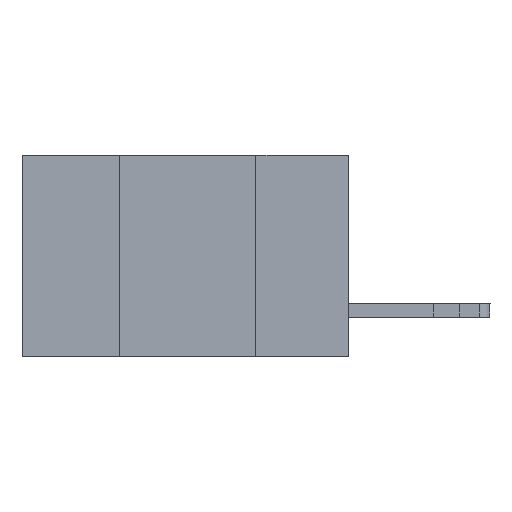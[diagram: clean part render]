
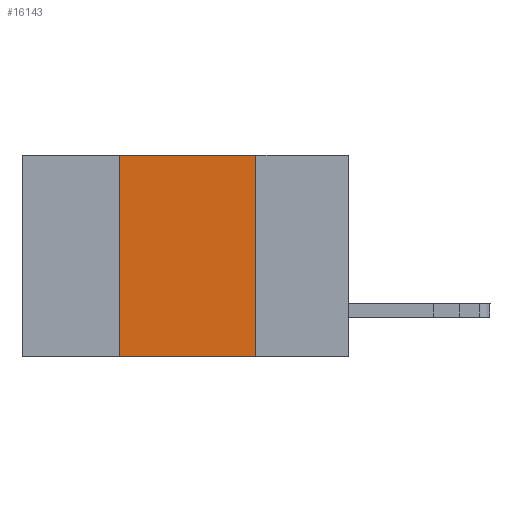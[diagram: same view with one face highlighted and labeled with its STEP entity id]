
A CAD part, left-side view. The second image highlights one B-rep face of the part: STEP entity #16143.
In plain terms, the highlighted planar face has unit normal (-1, 0, 0).
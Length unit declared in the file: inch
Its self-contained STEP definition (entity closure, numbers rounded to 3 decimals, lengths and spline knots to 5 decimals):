
#485 = AXIS2_PLACEMENT_3D ( 'NONE', #12607, #7604, #16830 ) ;
#1100 = EDGE_CURVE ( 'NONE', #4532, #9982, #6542, .T. ) ;
#1415 = ORIENTED_EDGE ( 'NONE', *, *, #6935, .F. ) ;
#1929 = VERTEX_POINT ( 'NONE', #5310 ) ;
#2057 = LINE ( 'NONE', #10616, #3103 ) ;
#2559 = LINE ( 'NONE', #4682, #4632 ) ;
#3103 = VECTOR ( 'NONE', #12013, 39.37008 ) ;
#3116 = EDGE_CURVE ( 'NONE', #1929, #9982, #2057, .T. ) ;
#3257 = LINE ( 'NONE', #12045, #14422 ) ;
#3979 = EDGE_LOOP ( 'NONE', ( #4754, #1415, #14849, #15293 ) ) ;
#4532 = VERTEX_POINT ( 'NONE', #10554 ) ;
#4632 = VECTOR ( 'NONE', #11650, 39.37008 ) ;
#4682 = CARTESIAN_POINT ( 'NONE',  ( 0., 0.6, 0. ) ) ;
#4754 = ORIENTED_EDGE ( 'NONE', *, *, #3116, .F. ) ;
#5310 = CARTESIAN_POINT ( 'NONE',  ( 0., 0.17, 0. ) ) ;
#6336 = CARTESIAN_POINT ( 'NONE',  ( 0., 0.17, -0.37 ) ) ;
#6542 = LINE ( 'NONE', #8313, #9777 ) ;
#6935 = EDGE_CURVE ( 'NONE', #13020, #1929, #2559, .T. ) ;
#7604 = DIRECTION ( 'NONE',  ( 1., 0., 0. ) ) ;
#8313 = CARTESIAN_POINT ( 'NONE',  ( 0., 0.6, -0.37 ) ) ;
#9777 = VECTOR ( 'NONE', #16618, 39.37008 ) ;
#9982 = VERTEX_POINT ( 'NONE', #6336 ) ;
#10554 = CARTESIAN_POINT ( 'NONE',  ( 0., 0.42, -0.37 ) ) ;
#10616 = CARTESIAN_POINT ( 'NONE',  ( 0., 0.17, 0. ) ) ;
#11650 = DIRECTION ( 'NONE',  ( 0., -1., 0. ) ) ;
#12013 = DIRECTION ( 'NONE',  ( 0., 0., -1. ) ) ;
#12045 = CARTESIAN_POINT ( 'NONE',  ( 0., 0.42, 0. ) ) ;
#12248 = FACE_OUTER_BOUND ( 'NONE', #3979, .T. ) ;
#12607 = CARTESIAN_POINT ( 'NONE',  ( 0., 0.6, 0. ) ) ;
#13020 = VERTEX_POINT ( 'NONE', #16695 ) ;
#13464 = DIRECTION ( 'NONE',  ( 0., 0., 1. ) ) ;
#14422 = VECTOR ( 'NONE', #13464, 39.37008 ) ;
#14849 = ORIENTED_EDGE ( 'NONE', *, *, #15129, .F. ) ;
#15129 = EDGE_CURVE ( 'NONE', #4532, #13020, #3257, .T. ) ;
#15293 = ORIENTED_EDGE ( 'NONE', *, *, #1100, .T. ) ;
#15491 = PLANE ( 'NONE',  #485 ) ;
#16143 = ADVANCED_FACE ( 'NONE', ( #12248 ), #15491, .F. ) ;
#16618 = DIRECTION ( 'NONE',  ( 0., -1., 0. ) ) ;
#16695 = CARTESIAN_POINT ( 'NONE',  ( 0., 0.42, 0. ) ) ;
#16830 = DIRECTION ( 'NONE',  ( 0., 0., -1. ) ) ;
